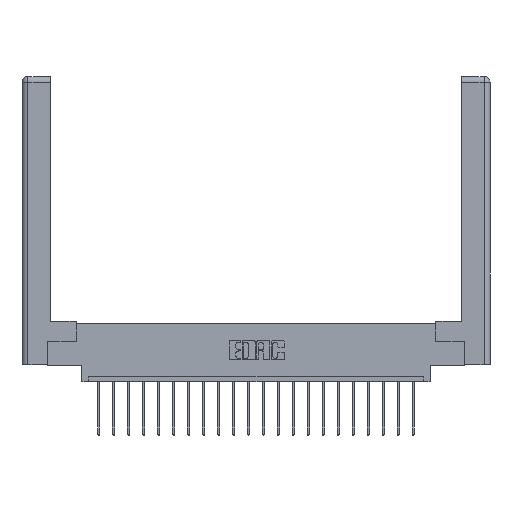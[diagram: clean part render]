
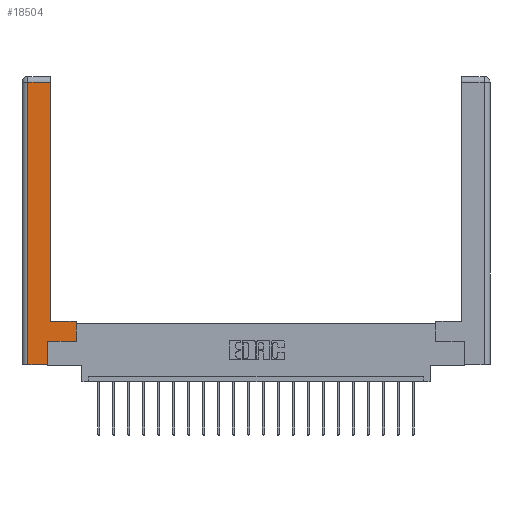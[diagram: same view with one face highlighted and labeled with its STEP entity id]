
A CAD part, top view. The second image highlights one B-rep face of the part: STEP entity #18504.
In plain terms, the highlighted planar face has unit normal (0, 0, 1).
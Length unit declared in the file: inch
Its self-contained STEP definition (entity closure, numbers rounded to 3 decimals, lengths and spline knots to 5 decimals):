
#907 = VECTOR ( 'NONE', #1113, 39.37008 ) ;
#1113 = DIRECTION ( 'NONE',  ( 0., -1., 0. ) ) ;
#1243 = EDGE_CURVE ( 'NONE', #12926, #15259, #9941, .T. ) ;
#1471 = CARTESIAN_POINT ( 'NONE',  ( 0., 0., 0. ) ) ;
#1948 = LINE ( 'NONE', #4743, #907 ) ;
#2108 = ORIENTED_EDGE ( 'NONE', *, *, #16027, .T. ) ;
#2708 = ORIENTED_EDGE ( 'NONE', *, *, #15308, .T. ) ;
#2824 = DIRECTION ( 'NONE',  ( 0., 1., 0. ) ) ;
#2951 = DIRECTION ( 'NONE',  ( 1., 0., 0. ) ) ;
#4152 = VERTEX_POINT ( 'NONE', #20919 ) ;
#4180 = VECTOR ( 'NONE', #8090, 39.37008 ) ;
#4196 = CARTESIAN_POINT ( 'NONE',  ( 0.295, 3., 0. ) ) ;
#4216 = VECTOR ( 'NONE', #2951, 39.37008 ) ;
#4220 = EDGE_CURVE ( 'NONE', #15259, #5453, #7430, .T. ) ;
#4501 = DIRECTION ( 'NONE',  ( 1., 0., 0. ) ) ;
#4593 = VECTOR ( 'NONE', #4501, 39.37008 ) ;
#4683 = PLANE ( 'NONE',  #16178 ) ;
#4743 = CARTESIAN_POINT ( 'NONE',  ( 0.0615, 0., 0. ) ) ;
#5453 = VERTEX_POINT ( 'NONE', #18175 ) ;
#6041 = LINE ( 'NONE', #9536, #4216 ) ;
#6169 = EDGE_CURVE ( 'NONE', #14566, #12926, #7036, .T. ) ;
#6357 = DIRECTION ( 'NONE',  ( -1., 0., 0. ) ) ;
#6386 = EDGE_LOOP ( 'NONE', ( #9361, #2708, #20060, #2108, #10271, #8837, #16226, #17705 ) ) ;
#6763 = CARTESIAN_POINT ( 'NONE',  ( 0.0615, 2.94, 0. ) ) ;
#6912 = VERTEX_POINT ( 'NONE', #19827 ) ;
#7036 = LINE ( 'NONE', #19699, #4180 ) ;
#7122 = CARTESIAN_POINT ( 'NONE',  ( 0.565, 0.45, 0. ) ) ;
#7430 = LINE ( 'NONE', #4196, #16137 ) ;
#7856 = CARTESIAN_POINT ( 'NONE',  ( 0.295, 0.45, 0. ) ) ;
#7992 = VECTOR ( 'NONE', #2824, 39.37008 ) ;
#8090 = DIRECTION ( 'NONE',  ( 0., 1., 0. ) ) ;
#8116 = DIRECTION ( 'NONE',  ( 0., 0., -1. ) ) ;
#8493 = CARTESIAN_POINT ( 'NONE',  ( 0.0615, 0., 0. ) ) ;
#8837 = ORIENTED_EDGE ( 'NONE', *, *, #13186, .T. ) ;
#9041 = LINE ( 'NONE', #13009, #4593 ) ;
#9296 = LINE ( 'NONE', #16183, #7992 ) ;
#9340 = VECTOR ( 'NONE', #14444, 39.37008 ) ;
#9361 = ORIENTED_EDGE ( 'NONE', *, *, #4220, .T. ) ;
#9536 = CARTESIAN_POINT ( 'NONE',  ( 0.565, 0.245, 0. ) ) ;
#9941 = LINE ( 'NONE', #7856, #13109 ) ;
#10271 = ORIENTED_EDGE ( 'NONE', *, *, #15926, .T. ) ;
#10524 = VERTEX_POINT ( 'NONE', #8493 ) ;
#10782 = DIRECTION ( 'NONE',  ( 0., 1., 0. ) ) ;
#12926 = VERTEX_POINT ( 'NONE', #7122 ) ;
#13009 = CARTESIAN_POINT ( 'NONE',  ( 0.265, 0., 0. ) ) ;
#13109 = VECTOR ( 'NONE', #14628, 39.37008 ) ;
#13186 = EDGE_CURVE ( 'NONE', #4152, #14566, #6041, .T. ) ;
#13611 = CARTESIAN_POINT ( 'NONE',  ( 0.565, 0.245, 0. ) ) ;
#14444 = DIRECTION ( 'NONE',  ( -1., 0., 0. ) ) ;
#14566 = VERTEX_POINT ( 'NONE', #13611 ) ;
#14628 = DIRECTION ( 'NONE',  ( -1., 0., 0. ) ) ;
#15259 = VERTEX_POINT ( 'NONE', #21113 ) ;
#15308 = EDGE_CURVE ( 'NONE', #5453, #19285, #19860, .T. ) ;
#15692 = FACE_OUTER_BOUND ( 'NONE', #6386, .T. ) ;
#15926 = EDGE_CURVE ( 'NONE', #6912, #4152, #9296, .T. ) ;
#15996 = CARTESIAN_POINT ( 'NONE',  ( 0.0615, 2.94, 0. ) ) ;
#16027 = EDGE_CURVE ( 'NONE', #10524, #6912, #9041, .T. ) ;
#16137 = VECTOR ( 'NONE', #10782, 39.37008 ) ;
#16178 = AXIS2_PLACEMENT_3D ( 'NONE', #1471, #8116, #6357 ) ;
#16183 = CARTESIAN_POINT ( 'NONE',  ( 0.265, 0.245, 0. ) ) ;
#16226 = ORIENTED_EDGE ( 'NONE', *, *, #6169, .T. ) ;
#17705 = ORIENTED_EDGE ( 'NONE', *, *, #1243, .T. ) ;
#18175 = CARTESIAN_POINT ( 'NONE',  ( 0.295, 2.94, 0. ) ) ;
#18504 = ADVANCED_FACE ( 'NONE', ( #15692 ), #4683, .F. ) ;
#19285 = VERTEX_POINT ( 'NONE', #6763 ) ;
#19699 = CARTESIAN_POINT ( 'NONE',  ( 0.565, 0.45, 0. ) ) ;
#19827 = CARTESIAN_POINT ( 'NONE',  ( 0.265, 0., 0. ) ) ;
#19860 = LINE ( 'NONE', #15996, #9340 ) ;
#20060 = ORIENTED_EDGE ( 'NONE', *, *, #20563, .T. ) ;
#20563 = EDGE_CURVE ( 'NONE', #19285, #10524, #1948, .T. ) ;
#20919 = CARTESIAN_POINT ( 'NONE',  ( 0.265, 0.245, 0. ) ) ;
#21113 = CARTESIAN_POINT ( 'NONE',  ( 0.295, 0.45, 0. ) ) ;
